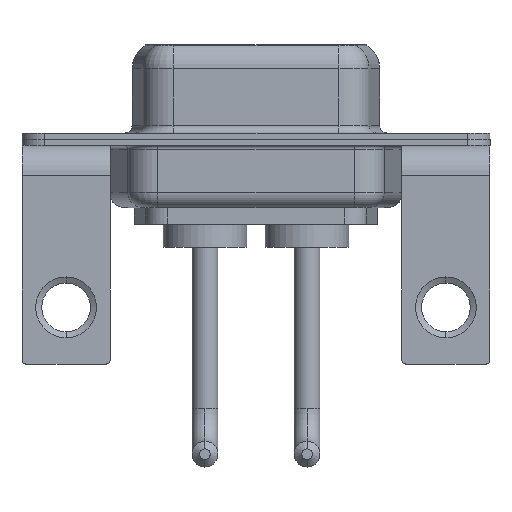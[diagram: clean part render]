
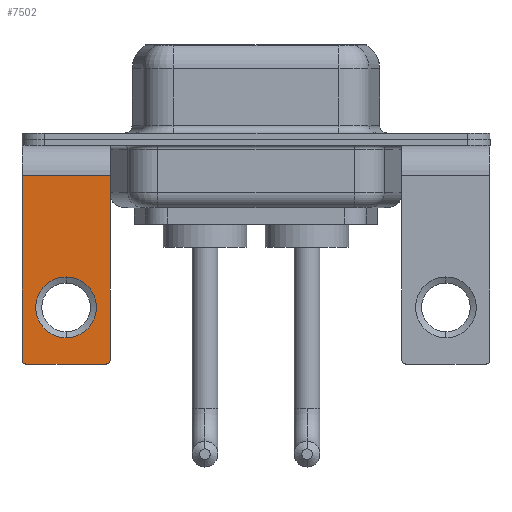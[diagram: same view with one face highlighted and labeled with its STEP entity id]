
A CAD part, front view. The second image highlights one B-rep face of the part: STEP entity #7502.
In plain terms, the highlighted planar face has unit normal (0, -1, 0).
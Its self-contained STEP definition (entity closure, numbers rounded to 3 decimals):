
#153 = VERTEX_POINT ( 'NONE', #12583 ) ;
#360 = CARTESIAN_POINT ( 'NONE',  ( 2.9, -6.25, -2.4 ) ) ;
#432 = DIRECTION ( 'NONE',  ( 0., 0., 1. ) ) ;
#469 = DIRECTION ( 'NONE',  ( -1., 0., 0. ) ) ;
#659 = EDGE_CURVE ( 'NONE', #6060, #1132, #12915, .T. ) ;
#747 = FACE_BOUND ( 'NONE', #7338, .T. ) ;
#774 = CARTESIAN_POINT ( 'NONE',  ( 2.9, -6.25, -2.4 ) ) ;
#1132 = VERTEX_POINT ( 'NONE', #8263 ) ;
#1265 = ORIENTED_EDGE ( 'NONE', *, *, #1535, .T. ) ;
#1516 = DIRECTION ( 'NONE',  ( 0., 0., 1. ) ) ;
#1535 = EDGE_CURVE ( 'NONE', #9303, #153, #2959, .T. ) ;
#1582 = VERTEX_POINT ( 'NONE', #4231 ) ;
#1657 = FACE_OUTER_BOUND ( 'NONE', #2867, .T. ) ;
#1975 = DIRECTION ( 'NONE',  ( -1., 0., 0. ) ) ;
#1983 = CARTESIAN_POINT ( 'NONE',  ( 2.9, -6.25, -14.8 ) ) ;
#2078 = DIRECTION ( 'NONE',  ( 0., 0., 1. ) ) ;
#2224 = AXIS2_PLACEMENT_3D ( 'NONE', #2839, #12771, #5775 ) ;
#2435 = DIRECTION ( 'NONE',  ( 0., 1., 0. ) ) ;
#2457 = VERTEX_POINT ( 'NONE', #11550 ) ;
#2572 = DIRECTION ( 'NONE',  ( 0., 0., -1. ) ) ;
#2581 = DIRECTION ( 'NONE',  ( 0., -1., 0. ) ) ;
#2597 = VERTEX_POINT ( 'NONE', #4019 ) ;
#2839 = CARTESIAN_POINT ( 'NONE',  ( 2.9, -6.25, -2.4 ) ) ;
#2867 = EDGE_LOOP ( 'NONE', ( #3139, #10564, #10465, #12607, #9636, #1265 ) ) ;
#2959 = LINE ( 'NONE', #6938, #8763 ) ;
#3138 = CIRCLE ( 'NONE', #8145, 2. ) ;
#3139 = ORIENTED_EDGE ( 'NONE', *, *, #11831, .T. ) ;
#3244 = CARTESIAN_POINT ( 'NONE',  ( 0., -6.25, -11.07 ) ) ;
#3288 = DIRECTION ( 'NONE',  ( 0., 0., -1. ) ) ;
#3341 = CIRCLE ( 'NONE', #7922, 2. ) ;
#3604 = VECTOR ( 'NONE', #3288, 1000. ) ;
#3921 = DIRECTION ( 'NONE',  ( 0., 1., 0. ) ) ;
#4019 = CARTESIAN_POINT ( 'NONE',  ( 0., -6.25, -9.07 ) ) ;
#4231 = CARTESIAN_POINT ( 'NONE',  ( 0., -6.25, -13.07 ) ) ;
#4275 = LINE ( 'NONE', #11149, #3604 ) ;
#4404 = EDGE_CURVE ( 'NONE', #1582, #2597, #3138, .T. ) ;
#5061 = AXIS2_PLACEMENT_3D ( 'NONE', #10984, #7033, #2078 ) ;
#5480 = CIRCLE ( 'NONE', #5061, 0.25 ) ;
#5775 = DIRECTION ( 'NONE',  ( 0., 0., 1. ) ) ;
#6060 = VERTEX_POINT ( 'NONE', #9315 ) ;
#6938 = CARTESIAN_POINT ( 'NONE',  ( 2.9, -6.25, -2.4 ) ) ;
#7033 = DIRECTION ( 'NONE',  ( 0., -1., 0. ) ) ;
#7196 = EDGE_CURVE ( 'NONE', #2597, #1582, #3341, .T. ) ;
#7338 = EDGE_LOOP ( 'NONE', ( #11289, #10065 ) ) ;
#7464 = AXIS2_PLACEMENT_3D ( 'NONE', #12523, #2581, #432 ) ;
#7490 = EDGE_CURVE ( 'NONE', #9303, #8212, #11545, .T. ) ;
#7502 = ADVANCED_FACE ( 'NONE', ( #747, #1657 ), #11815, .F. ) ;
#7544 = VECTOR ( 'NONE', #469, 1000. ) ;
#7838 = EDGE_CURVE ( 'NONE', #2457, #1132, #10957, .T. ) ;
#7922 = AXIS2_PLACEMENT_3D ( 'NONE', #3244, #3921, #12278 ) ;
#8145 = AXIS2_PLACEMENT_3D ( 'NONE', #10545, #2435, #1516 ) ;
#8212 = VERTEX_POINT ( 'NONE', #11929 ) ;
#8263 = CARTESIAN_POINT ( 'NONE',  ( -2.65, -6.25, -14.8 ) ) ;
#8763 = VECTOR ( 'NONE', #1975, 1000. ) ;
#9303 = VERTEX_POINT ( 'NONE', #774 ) ;
#9315 = CARTESIAN_POINT ( 'NONE',  ( -2.9, -6.25, -14.55 ) ) ;
#9587 = EDGE_CURVE ( 'NONE', #2457, #8212, #5480, .T. ) ;
#9636 = ORIENTED_EDGE ( 'NONE', *, *, #7490, .F. ) ;
#9974 = VECTOR ( 'NONE', #2572, 1000. ) ;
#10065 = ORIENTED_EDGE ( 'NONE', *, *, #7196, .T. ) ;
#10465 = ORIENTED_EDGE ( 'NONE', *, *, #7838, .F. ) ;
#10545 = CARTESIAN_POINT ( 'NONE',  ( 0., -6.25, -11.07 ) ) ;
#10564 = ORIENTED_EDGE ( 'NONE', *, *, #659, .T. ) ;
#10957 = LINE ( 'NONE', #1983, #7544 ) ;
#10984 = CARTESIAN_POINT ( 'NONE',  ( 2.65, -6.25, -14.55 ) ) ;
#11149 = CARTESIAN_POINT ( 'NONE',  ( -2.9, -6.25, -2.4 ) ) ;
#11289 = ORIENTED_EDGE ( 'NONE', *, *, #4404, .T. ) ;
#11545 = LINE ( 'NONE', #360, #9974 ) ;
#11550 = CARTESIAN_POINT ( 'NONE',  ( 2.65, -6.25, -14.8 ) ) ;
#11815 = PLANE ( 'NONE',  #2224 ) ;
#11831 = EDGE_CURVE ( 'NONE', #153, #6060, #4275, .T. ) ;
#11929 = CARTESIAN_POINT ( 'NONE',  ( 2.9, -6.25, -14.55 ) ) ;
#12278 = DIRECTION ( 'NONE',  ( 0., 0., 1. ) ) ;
#12523 = CARTESIAN_POINT ( 'NONE',  ( -2.65, -6.25, -14.55 ) ) ;
#12583 = CARTESIAN_POINT ( 'NONE',  ( -2.9, -6.25, -2.4 ) ) ;
#12607 = ORIENTED_EDGE ( 'NONE', *, *, #9587, .T. ) ;
#12771 = DIRECTION ( 'NONE',  ( 0., 1., 0. ) ) ;
#12915 = CIRCLE ( 'NONE', #7464, 0.25 ) ;
